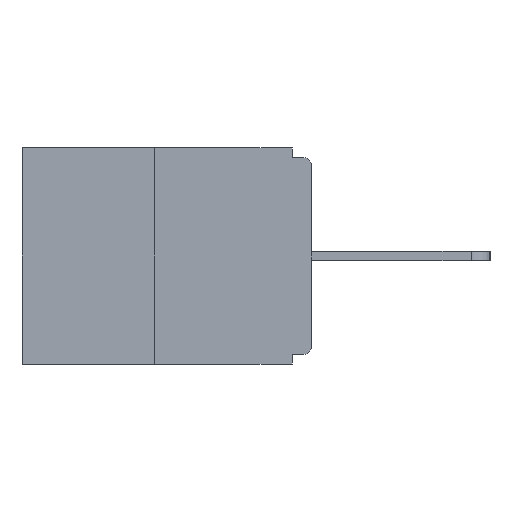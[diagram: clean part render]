
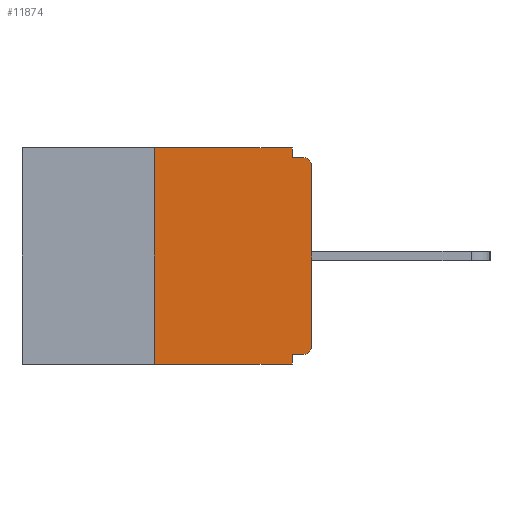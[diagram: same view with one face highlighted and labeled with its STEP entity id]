
A CAD part, left-side view. The second image highlights one B-rep face of the part: STEP entity #11874.
In plain terms, the highlighted planar face has unit normal (-1, 0, 0).
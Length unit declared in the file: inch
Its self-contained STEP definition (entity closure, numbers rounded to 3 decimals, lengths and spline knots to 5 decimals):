
#42 = LINE ( 'NONE', #20378, #5047 ) ;
#721 = CARTESIAN_POINT ( 'NONE',  ( 0., 0.031, -0.015 ) ) ;
#861 = CARTESIAN_POINT ( 'NONE',  ( 0., 0., -0.328 ) ) ;
#923 = CIRCLE ( 'NONE', #20816, 0.015 ) ;
#1336 = CARTESIAN_POINT ( 'NONE',  ( 0., 0.46, 0. ) ) ;
#1497 = VERTEX_POINT ( 'NONE', #13818 ) ;
#2166 = CIRCLE ( 'NONE', #6772, 0.015 ) ;
#2478 = DIRECTION ( 'NONE',  ( 0., -1., 0. ) ) ;
#2974 = EDGE_LOOP ( 'NONE', ( #4167, #23849, #23121, #11640, #11748, #14395, #8741, #10887, #16435, #13756 ) ) ;
#3428 = DIRECTION ( 'NONE',  ( 0., 0., -1. ) ) ;
#3444 = DIRECTION ( 'NONE',  ( -1., 0., 0. ) ) ;
#3731 = VECTOR ( 'NONE', #23020, 39.37008 ) ;
#4167 = ORIENTED_EDGE ( 'NONE', *, *, #24675, .F. ) ;
#4614 = DIRECTION ( 'NONE',  ( 0., 0., 1. ) ) ;
#5047 = VECTOR ( 'NONE', #10345, 39.37008 ) ;
#5200 = VERTEX_POINT ( 'NONE', #721 ) ;
#5211 = CARTESIAN_POINT ( 'NONE',  ( 0., 0., -0.015 ) ) ;
#5458 = EDGE_CURVE ( 'NONE', #14541, #15135, #11315, .T. ) ;
#6097 = CARTESIAN_POINT ( 'NONE',  ( 0., 0.46, -0.343 ) ) ;
#6244 = LINE ( 'NONE', #5211, #3731 ) ;
#6378 = FACE_OUTER_BOUND ( 'NONE', #2974, .T. ) ;
#6663 = CARTESIAN_POINT ( 'NONE',  ( 0., 0.031, -0.343 ) ) ;
#6693 = LINE ( 'NONE', #19038, #24690 ) ;
#6772 = AXIS2_PLACEMENT_3D ( 'NONE', #10922, #3444, #23417 ) ;
#7472 = VERTEX_POINT ( 'NONE', #17710 ) ;
#7791 = VECTOR ( 'NONE', #2478, 39.37008 ) ;
#8679 = AXIS2_PLACEMENT_3D ( 'NONE', #1336, #21666, #3428 ) ;
#8741 = ORIENTED_EDGE ( 'NONE', *, *, #14575, .T. ) ;
#9626 = CARTESIAN_POINT ( 'NONE',  ( 0., 0.031, -0.343 ) ) ;
#9848 = EDGE_CURVE ( 'NONE', #17142, #26045, #923, .T. ) ;
#10345 = DIRECTION ( 'NONE',  ( 0., 0., -1. ) ) ;
#10582 = CARTESIAN_POINT ( 'NONE',  ( 0., 0.031, -0.328 ) ) ;
#10887 = ORIENTED_EDGE ( 'NONE', *, *, #9848, .T. ) ;
#10922 = CARTESIAN_POINT ( 'NONE',  ( 0., 0.015, -0.313 ) ) ;
#11182 = EDGE_CURVE ( 'NONE', #17895, #7472, #24939, .T. ) ;
#11262 = LINE ( 'NONE', #24832, #16873 ) ;
#11315 = LINE ( 'NONE', #861, #21404 ) ;
#11348 = VECTOR ( 'NONE', #20755, 39.37008 ) ;
#11640 = ORIENTED_EDGE ( 'NONE', *, *, #18129, .F. ) ;
#11748 = ORIENTED_EDGE ( 'NONE', *, *, #5458, .F. ) ;
#11874 = ADVANCED_FACE ( 'NONE', ( #6378 ), #17226, .F. ) ;
#12260 = CARTESIAN_POINT ( 'NONE',  ( 0., 0.25, -0.343 ) ) ;
#12835 = DIRECTION ( 'NONE',  ( 0., -1., 0. ) ) ;
#13015 = EDGE_CURVE ( 'NONE', #16881, #5200, #42, .T. ) ;
#13756 = ORIENTED_EDGE ( 'NONE', *, *, #13015, .F. ) ;
#13818 = CARTESIAN_POINT ( 'NONE',  ( 0., 0., -0.313 ) ) ;
#14395 = ORIENTED_EDGE ( 'NONE', *, *, #16969, .T. ) ;
#14541 = VERTEX_POINT ( 'NONE', #14587 ) ;
#14575 = EDGE_CURVE ( 'NONE', #1497, #17142, #6693, .T. ) ;
#14587 = CARTESIAN_POINT ( 'NONE',  ( 0., 0.015, -0.328 ) ) ;
#14711 = DIRECTION ( 'NONE',  ( -1., 0., 0. ) ) ;
#14730 = LINE ( 'NONE', #6097, #7791 ) ;
#15135 = VERTEX_POINT ( 'NONE', #10582 ) ;
#16379 = CARTESIAN_POINT ( 'NONE',  ( 0., 0.015, -0.015 ) ) ;
#16435 = ORIENTED_EDGE ( 'NONE', *, *, #20130, .F. ) ;
#16830 = CARTESIAN_POINT ( 'NONE',  ( 0., 0.25, 0. ) ) ;
#16873 = VECTOR ( 'NONE', #12835, 39.37008 ) ;
#16881 = VERTEX_POINT ( 'NONE', #20780 ) ;
#16969 = EDGE_CURVE ( 'NONE', #14541, #1497, #2166, .T. ) ;
#17142 = VERTEX_POINT ( 'NONE', #20229 ) ;
#17226 = PLANE ( 'NONE',  #8679 ) ;
#17710 = CARTESIAN_POINT ( 'NONE',  ( 0., 0.25, 0. ) ) ;
#17895 = VERTEX_POINT ( 'NONE', #12260 ) ;
#18129 = EDGE_CURVE ( 'NONE', #15135, #21658, #19847, .T. ) ;
#18723 = CARTESIAN_POINT ( 'NONE',  ( 0., 0.015, -0.03 ) ) ;
#19038 = CARTESIAN_POINT ( 'NONE',  ( 0., 0., 0. ) ) ;
#19847 = LINE ( 'NONE', #6663, #11348 ) ;
#20130 = EDGE_CURVE ( 'NONE', #5200, #26045, #6244, .T. ) ;
#20229 = CARTESIAN_POINT ( 'NONE',  ( 0., 0., -0.03 ) ) ;
#20378 = CARTESIAN_POINT ( 'NONE',  ( 0., 0.031, 0. ) ) ;
#20452 = EDGE_CURVE ( 'NONE', #17895, #21658, #14730, .T. ) ;
#20755 = DIRECTION ( 'NONE',  ( 0., 0., -1. ) ) ;
#20780 = CARTESIAN_POINT ( 'NONE',  ( 0., 0.031, 0. ) ) ;
#20816 = AXIS2_PLACEMENT_3D ( 'NONE', #18723, #14711, #23095 ) ;
#21125 = DIRECTION ( 'NONE',  ( 0., 0., 1. ) ) ;
#21404 = VECTOR ( 'NONE', #25050, 39.37008 ) ;
#21658 = VERTEX_POINT ( 'NONE', #9626 ) ;
#21666 = DIRECTION ( 'NONE',  ( 1., 0., 0. ) ) ;
#23020 = DIRECTION ( 'NONE',  ( 0., -1., 0. ) ) ;
#23095 = DIRECTION ( 'NONE',  ( 0., 0., -1. ) ) ;
#23121 = ORIENTED_EDGE ( 'NONE', *, *, #20452, .T. ) ;
#23417 = DIRECTION ( 'NONE',  ( 0., 0., -1. ) ) ;
#23849 = ORIENTED_EDGE ( 'NONE', *, *, #11182, .F. ) ;
#24309 = VECTOR ( 'NONE', #4614, 39.37008 ) ;
#24675 = EDGE_CURVE ( 'NONE', #7472, #16881, #11262, .T. ) ;
#24690 = VECTOR ( 'NONE', #21125, 39.37008 ) ;
#24832 = CARTESIAN_POINT ( 'NONE',  ( 0., 0.46, 0. ) ) ;
#24939 = LINE ( 'NONE', #16830, #24309 ) ;
#25050 = DIRECTION ( 'NONE',  ( 0., 1., 0. ) ) ;
#26045 = VERTEX_POINT ( 'NONE', #16379 ) ;
